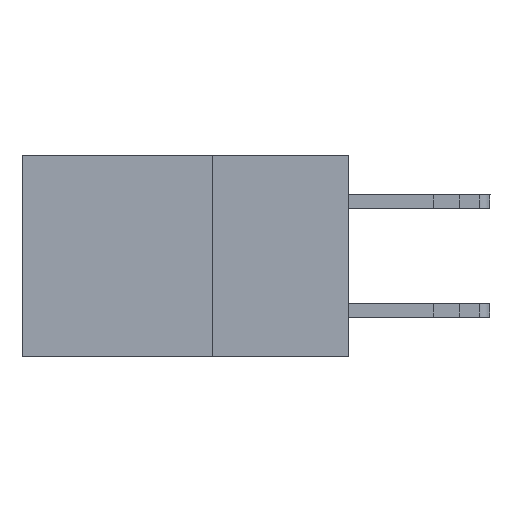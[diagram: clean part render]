
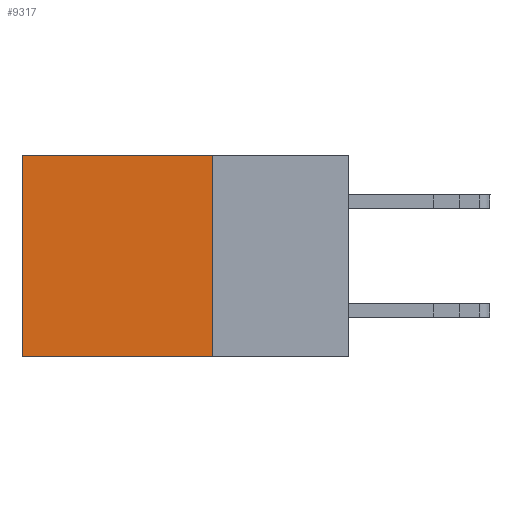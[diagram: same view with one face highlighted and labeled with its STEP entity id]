
A CAD part, left-side view. The second image highlights one B-rep face of the part: STEP entity #9317.
In plain terms, the highlighted planar face has unit normal (-1, 0, 0).
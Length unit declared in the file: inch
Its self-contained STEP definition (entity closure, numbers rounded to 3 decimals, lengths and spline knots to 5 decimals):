
#2638 = DIRECTION ( 'NONE',  ( 0., 0., -1. ) ) ;
#3306 = VERTEX_POINT ( 'NONE', #17340 ) ;
#4071 = CARTESIAN_POINT ( 'NONE',  ( 0.298, 0.25, -0.37 ) ) ;
#4486 = FACE_OUTER_BOUND ( 'NONE', #16407, .T. ) ;
#6383 = VECTOR ( 'NONE', #19801, 39.37008 ) ;
#6452 = CARTESIAN_POINT ( 'NONE',  ( 0.298, 0.25, -0.37 ) ) ;
#7109 = CARTESIAN_POINT ( 'NONE',  ( 0.298, 0.25, 0. ) ) ;
#7457 = ORIENTED_EDGE ( 'NONE', *, *, #18272, .F. ) ;
#7863 = PLANE ( 'NONE',  #22678 ) ;
#8199 = LINE ( 'NONE', #6452, #11166 ) ;
#8312 = CARTESIAN_POINT ( 'NONE',  ( 0.298, 0.25, 0. ) ) ;
#9003 = EDGE_CURVE ( 'NONE', #9265, #10471, #13208, .T. ) ;
#9265 = VERTEX_POINT ( 'NONE', #8312 ) ;
#9317 = ADVANCED_FACE ( 'NONE', ( #4486 ), #7863, .F. ) ;
#9396 = CARTESIAN_POINT ( 'NONE',  ( 0.298, 0.6, 0. ) ) ;
#9952 = ORIENTED_EDGE ( 'NONE', *, *, #9003, .F. ) ;
#10355 = VECTOR ( 'NONE', #14142, 39.37008 ) ;
#10471 = VERTEX_POINT ( 'NONE', #4071 ) ;
#11166 = VECTOR ( 'NONE', #19992, 39.37008 ) ;
#11484 = CARTESIAN_POINT ( 'NONE',  ( 0.298, 0.25, 0. ) ) ;
#13208 = LINE ( 'NONE', #11484, #15667 ) ;
#13277 = DIRECTION ( 'NONE',  ( 1., 0., 0. ) ) ;
#14142 = DIRECTION ( 'NONE',  ( 0., 1., 0. ) ) ;
#14358 = EDGE_CURVE ( 'NONE', #9265, #16806, #21310, .T. ) ;
#15667 = VECTOR ( 'NONE', #20262, 39.37008 ) ;
#16407 = EDGE_LOOP ( 'NONE', ( #19271, #7457, #9952, #22519 ) ) ;
#16785 = LINE ( 'NONE', #9396, #6383 ) ;
#16806 = VERTEX_POINT ( 'NONE', #17234 ) ;
#17234 = CARTESIAN_POINT ( 'NONE',  ( 0.298, 0.6, 0. ) ) ;
#17340 = CARTESIAN_POINT ( 'NONE',  ( 0.298, 0.6, -0.37 ) ) ;
#18272 = EDGE_CURVE ( 'NONE', #10471, #3306, #8199, .T. ) ;
#19271 = ORIENTED_EDGE ( 'NONE', *, *, #19538, .T. ) ;
#19538 = EDGE_CURVE ( 'NONE', #16806, #3306, #16785, .T. ) ;
#19801 = DIRECTION ( 'NONE',  ( 0., 0., -1. ) ) ;
#19992 = DIRECTION ( 'NONE',  ( 0., 1., 0. ) ) ;
#20262 = DIRECTION ( 'NONE',  ( 0., 0., -1. ) ) ;
#21310 = LINE ( 'NONE', #7109, #10355 ) ;
#22054 = CARTESIAN_POINT ( 'NONE',  ( 0.298, 0.25, 0. ) ) ;
#22519 = ORIENTED_EDGE ( 'NONE', *, *, #14358, .T. ) ;
#22678 = AXIS2_PLACEMENT_3D ( 'NONE', #22054, #13277, #2638 ) ;
